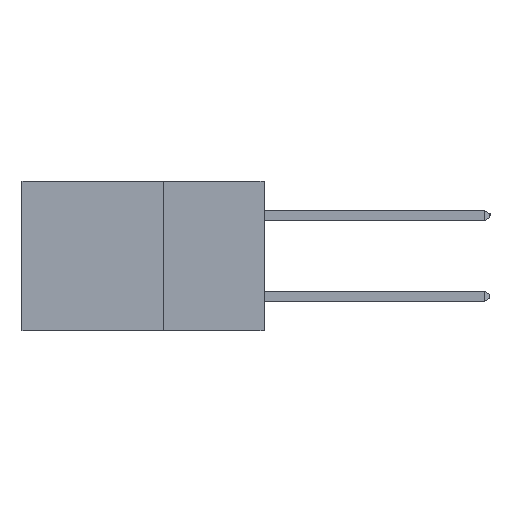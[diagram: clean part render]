
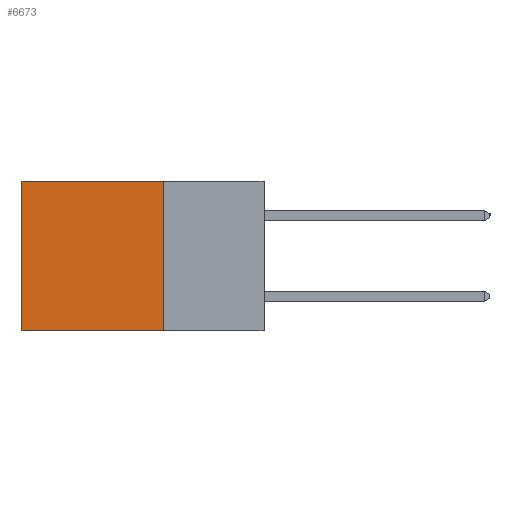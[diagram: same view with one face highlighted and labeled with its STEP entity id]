
A CAD part, left-side view. The second image highlights one B-rep face of the part: STEP entity #6673.
In plain terms, the highlighted planar face has unit normal (-1, 0, 0).
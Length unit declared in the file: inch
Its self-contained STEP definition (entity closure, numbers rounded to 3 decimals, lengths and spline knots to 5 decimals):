
#121 = DIRECTION ( 'NONE',  ( 1., 0., 0. ) ) ;
#521 = EDGE_CURVE ( 'NONE', #5928, #11292, #7404, .T. ) ;
#924 = CARTESIAN_POINT ( 'NONE',  ( 0.2615, 0.6, -0.37 ) ) ;
#988 = CARTESIAN_POINT ( 'NONE',  ( 0.2615, 0.6, -0.37 ) ) ;
#1022 = CARTESIAN_POINT ( 'NONE',  ( 0.2615, 0.25, 0. ) ) ;
#1175 = VECTOR ( 'NONE', #5337, 39.37008 ) ;
#1180 = ORIENTED_EDGE ( 'NONE', *, *, #5383, .F. ) ;
#1368 = CARTESIAN_POINT ( 'NONE',  ( 0.2615, 0.25, -0.37 ) ) ;
#1393 = VERTEX_POINT ( 'NONE', #1022 ) ;
#1398 = LINE ( 'NONE', #9124, #13784 ) ;
#1767 = CARTESIAN_POINT ( 'NONE',  ( 0.2615, 0.6, 0. ) ) ;
#1837 = VERTEX_POINT ( 'NONE', #9109 ) ;
#1978 = ORIENTED_EDGE ( 'NONE', *, *, #521, .T. ) ;
#3537 = DIRECTION ( 'NONE',  ( 0., 0., -1. ) ) ;
#4109 = VECTOR ( 'NONE', #3537, 39.37008 ) ;
#5337 = DIRECTION ( 'NONE',  ( 0., 0., -1. ) ) ;
#5383 = EDGE_CURVE ( 'NONE', #1393, #1837, #6720, .T. ) ;
#5645 = ORIENTED_EDGE ( 'NONE', *, *, #10070, .T. ) ;
#5928 = VERTEX_POINT ( 'NONE', #1767 ) ;
#6137 = EDGE_LOOP ( 'NONE', ( #1978, #8000, #1180, #5645 ) ) ;
#6527 = PLANE ( 'NONE',  #12873 ) ;
#6673 = ADVANCED_FACE ( 'NONE', ( #12133 ), #6527, .F. ) ;
#6720 = LINE ( 'NONE', #1368, #4109 ) ;
#7404 = LINE ( 'NONE', #924, #1175 ) ;
#7612 = DIRECTION ( 'NONE',  ( 0., 1., 0. ) ) ;
#8000 = ORIENTED_EDGE ( 'NONE', *, *, #13853, .F. ) ;
#8125 = CARTESIAN_POINT ( 'NONE',  ( 0.2615, 0.25, -0.37 ) ) ;
#9109 = CARTESIAN_POINT ( 'NONE',  ( 0.2615, 0.25, -0.37 ) ) ;
#9124 = CARTESIAN_POINT ( 'NONE',  ( 0.2615, 0.25, 0. ) ) ;
#9690 = CARTESIAN_POINT ( 'NONE',  ( 0.2615, 0.25, -0.37 ) ) ;
#10070 = EDGE_CURVE ( 'NONE', #1393, #5928, #1398, .T. ) ;
#10225 = LINE ( 'NONE', #8125, #10962 ) ;
#10790 = DIRECTION ( 'NONE',  ( 0., 0., -1. ) ) ;
#10962 = VECTOR ( 'NONE', #11336, 39.37008 ) ;
#11292 = VERTEX_POINT ( 'NONE', #988 ) ;
#11336 = DIRECTION ( 'NONE',  ( 0., 1., 0. ) ) ;
#12133 = FACE_OUTER_BOUND ( 'NONE', #6137, .T. ) ;
#12873 = AXIS2_PLACEMENT_3D ( 'NONE', #9690, #121, #10790 ) ;
#13784 = VECTOR ( 'NONE', #7612, 39.37008 ) ;
#13853 = EDGE_CURVE ( 'NONE', #1837, #11292, #10225, .T. ) ;
